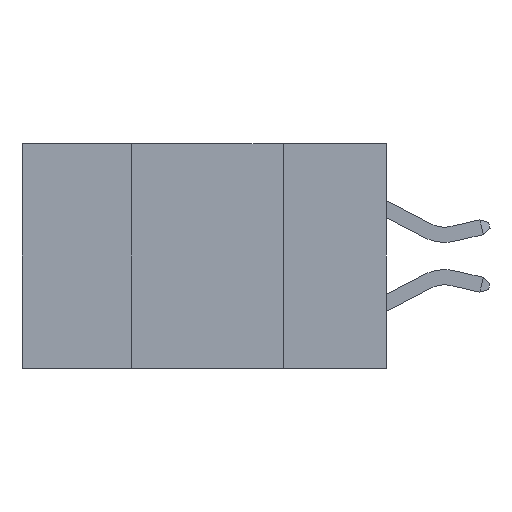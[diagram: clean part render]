
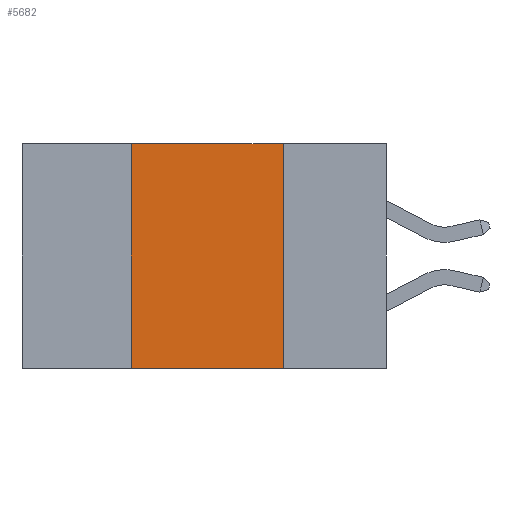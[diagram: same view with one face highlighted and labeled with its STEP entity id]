
A CAD part, left-side view. The second image highlights one B-rep face of the part: STEP entity #5682.
In plain terms, the highlighted planar face has unit normal (-1, 0, 0).
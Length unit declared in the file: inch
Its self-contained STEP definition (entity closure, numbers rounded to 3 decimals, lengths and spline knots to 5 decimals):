
#138 = DIRECTION ( 'NONE',  ( 0., 0., -1. ) ) ;
#677 = LINE ( 'NONE', #5484, #3889 ) ;
#938 = CARTESIAN_POINT ( 'NONE',  ( 0., 0.17, -0.37 ) ) ;
#1692 = EDGE_LOOP ( 'NONE', ( #3052, #4890, #11378, #2572 ) ) ;
#1807 = VERTEX_POINT ( 'NONE', #3250 ) ;
#2175 = VECTOR ( 'NONE', #4801, 39.37008 ) ;
#2516 = CARTESIAN_POINT ( 'NONE',  ( 0., 0.42, -0.37 ) ) ;
#2556 = VECTOR ( 'NONE', #9513, 39.37008 ) ;
#2572 = ORIENTED_EDGE ( 'NONE', *, *, #9097, .T. ) ;
#3052 = ORIENTED_EDGE ( 'NONE', *, *, #11741, .F. ) ;
#3207 = VERTEX_POINT ( 'NONE', #4606 ) ;
#3250 = CARTESIAN_POINT ( 'NONE',  ( 0., 0.42, 0. ) ) ;
#3889 = VECTOR ( 'NONE', #10350, 39.37008 ) ;
#4052 = CARTESIAN_POINT ( 'NONE',  ( 0., 0.6, 0. ) ) ;
#4121 = DIRECTION ( 'NONE',  ( 1., 0., 0. ) ) ;
#4606 = CARTESIAN_POINT ( 'NONE',  ( 0., 0.17, 0. ) ) ;
#4801 = DIRECTION ( 'NONE',  ( 0., 0., -1. ) ) ;
#4890 = ORIENTED_EDGE ( 'NONE', *, *, #11240, .F. ) ;
#5484 = CARTESIAN_POINT ( 'NONE',  ( 0., 0.6, -0.37 ) ) ;
#5669 = CARTESIAN_POINT ( 'NONE',  ( 0., 0.6, 0. ) ) ;
#5682 = ADVANCED_FACE ( 'NONE', ( #7052 ), #6027, .F. ) ;
#5900 = EDGE_CURVE ( 'NONE', #8151, #1807, #7348, .T. ) ;
#6027 = PLANE ( 'NONE',  #11489 ) ;
#7052 = FACE_OUTER_BOUND ( 'NONE', #1692, .T. ) ;
#7231 = DIRECTION ( 'NONE',  ( 0., 0., 1. ) ) ;
#7348 = LINE ( 'NONE', #2516, #8861 ) ;
#8151 = VERTEX_POINT ( 'NONE', #10616 ) ;
#8480 = VERTEX_POINT ( 'NONE', #11786 ) ;
#8495 = LINE ( 'NONE', #5669, #2556 ) ;
#8861 = VECTOR ( 'NONE', #7231, 39.37008 ) ;
#9097 = EDGE_CURVE ( 'NONE', #8151, #8480, #677, .T. ) ;
#9513 = DIRECTION ( 'NONE',  ( 0., -1., 0. ) ) ;
#9600 = LINE ( 'NONE', #938, #2175 ) ;
#10350 = DIRECTION ( 'NONE',  ( 0., -1., 0. ) ) ;
#10616 = CARTESIAN_POINT ( 'NONE',  ( 0., 0.42, -0.37 ) ) ;
#11240 = EDGE_CURVE ( 'NONE', #1807, #3207, #8495, .T. ) ;
#11378 = ORIENTED_EDGE ( 'NONE', *, *, #5900, .F. ) ;
#11489 = AXIS2_PLACEMENT_3D ( 'NONE', #4052, #4121, #138 ) ;
#11741 = EDGE_CURVE ( 'NONE', #3207, #8480, #9600, .T. ) ;
#11786 = CARTESIAN_POINT ( 'NONE',  ( 0., 0.17, -0.37 ) ) ;
